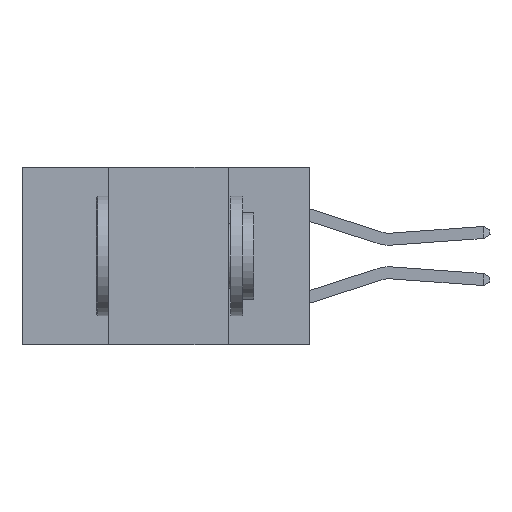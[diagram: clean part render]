
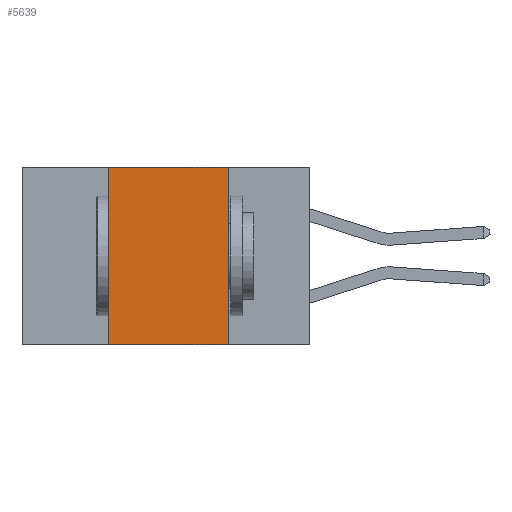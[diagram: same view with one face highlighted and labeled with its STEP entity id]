
A CAD part, left-side view. The second image highlights one B-rep face of the part: STEP entity #5639.
In plain terms, the highlighted planar face has unit normal (-1, 0, 0).
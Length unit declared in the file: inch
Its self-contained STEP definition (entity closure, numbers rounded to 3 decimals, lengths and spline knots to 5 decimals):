
#468 = CARTESIAN_POINT ( 'NONE',  ( 0., 0.6, 0. ) ) ;
#579 = DIRECTION ( 'NONE',  ( 0., 0., -1. ) ) ;
#581 = EDGE_CURVE ( 'NONE', #3124, #8581, #6055, .T. ) ;
#1177 = EDGE_CURVE ( 'NONE', #3124, #2705, #8674, .T. ) ;
#1368 = DIRECTION ( 'NONE',  ( 0., 0., -1. ) ) ;
#1748 = CARTESIAN_POINT ( 'NONE',  ( 0., 0.17, -0.37 ) ) ;
#1779 = EDGE_CURVE ( 'NONE', #2705, #4379, #1921, .T. ) ;
#1845 = ORIENTED_EDGE ( 'NONE', *, *, #1177, .F. ) ;
#1921 = LINE ( 'NONE', #10423, #6900 ) ;
#2350 = VECTOR ( 'NONE', #579, 39.37008 ) ;
#2414 = EDGE_CURVE ( 'NONE', #4379, #8581, #9524, .T. ) ;
#2705 = VERTEX_POINT ( 'NONE', #3940 ) ;
#3124 = VERTEX_POINT ( 'NONE', #7642 ) ;
#3472 = CARTESIAN_POINT ( 'NONE',  ( 0., 0.42, -0.37 ) ) ;
#3940 = CARTESIAN_POINT ( 'NONE',  ( 0., 0.42, 0. ) ) ;
#4041 = ORIENTED_EDGE ( 'NONE', *, *, #581, .T. ) ;
#4379 = VERTEX_POINT ( 'NONE', #4666 ) ;
#4666 = CARTESIAN_POINT ( 'NONE',  ( 0., 0.17, 0. ) ) ;
#5639 = ADVANCED_FACE ( 'NONE', ( #8604 ), #11574, .F. ) ;
#5739 = DIRECTION ( 'NONE',  ( 0., -1., 0. ) ) ;
#6055 = LINE ( 'NONE', #8623, #8263 ) ;
#6178 = VECTOR ( 'NONE', #9931, 39.37008 ) ;
#6818 = ORIENTED_EDGE ( 'NONE', *, *, #1779, .F. ) ;
#6888 = AXIS2_PLACEMENT_3D ( 'NONE', #468, #6958, #1368 ) ;
#6900 = VECTOR ( 'NONE', #11119, 39.37008 ) ;
#6958 = DIRECTION ( 'NONE',  ( 1., 0., 0. ) ) ;
#7642 = CARTESIAN_POINT ( 'NONE',  ( 0., 0.42, -0.37 ) ) ;
#7666 = EDGE_LOOP ( 'NONE', ( #9311, #6818, #1845, #4041 ) ) ;
#7703 = CARTESIAN_POINT ( 'NONE',  ( 0., 0.17, -0.37 ) ) ;
#8263 = VECTOR ( 'NONE', #5739, 39.37008 ) ;
#8581 = VERTEX_POINT ( 'NONE', #7703 ) ;
#8604 = FACE_OUTER_BOUND ( 'NONE', #7666, .T. ) ;
#8623 = CARTESIAN_POINT ( 'NONE',  ( 0., 0.6, -0.37 ) ) ;
#8674 = LINE ( 'NONE', #3472, #6178 ) ;
#9311 = ORIENTED_EDGE ( 'NONE', *, *, #2414, .F. ) ;
#9524 = LINE ( 'NONE', #1748, #2350 ) ;
#9931 = DIRECTION ( 'NONE',  ( 0., 0., 1. ) ) ;
#10423 = CARTESIAN_POINT ( 'NONE',  ( 0., 0.6, 0. ) ) ;
#11119 = DIRECTION ( 'NONE',  ( 0., -1., 0. ) ) ;
#11574 = PLANE ( 'NONE',  #6888 ) ;
